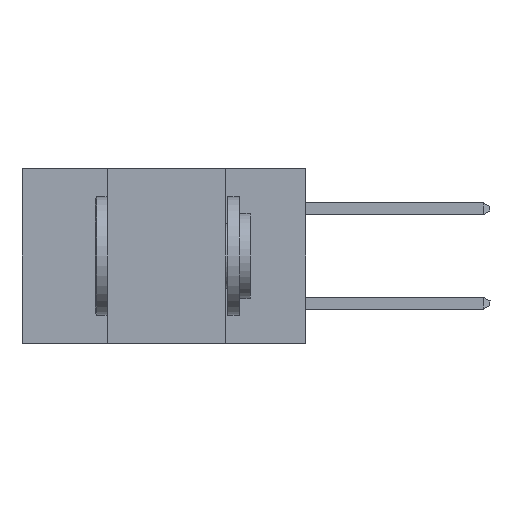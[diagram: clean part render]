
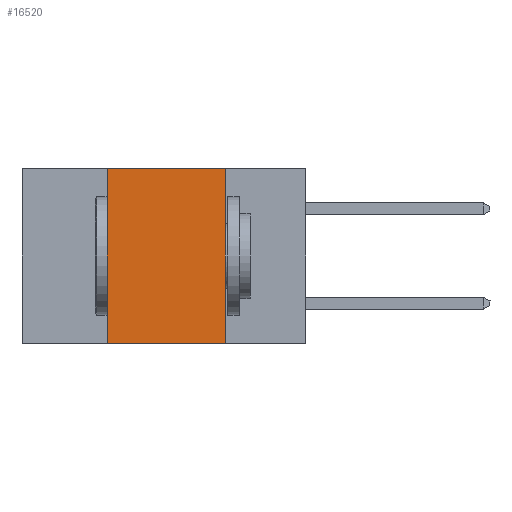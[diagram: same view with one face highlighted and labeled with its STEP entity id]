
A CAD part, left-side view. The second image highlights one B-rep face of the part: STEP entity #16520.
In plain terms, the highlighted planar face has unit normal (-1, 0, 0).
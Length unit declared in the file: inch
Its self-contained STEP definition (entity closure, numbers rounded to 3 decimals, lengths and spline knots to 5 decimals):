
#787 = CARTESIAN_POINT ( 'NONE',  ( 0., 0.42, -0.37 ) ) ;
#958 = CARTESIAN_POINT ( 'NONE',  ( 0., 0.17, 0. ) ) ;
#2046 = ORIENTED_EDGE ( 'NONE', *, *, #6565, .F. ) ;
#2232 = ORIENTED_EDGE ( 'NONE', *, *, #5936, .F. ) ;
#3560 = CARTESIAN_POINT ( 'NONE',  ( 0., 0.42, 0. ) ) ;
#4858 = PLANE ( 'NONE',  #14725 ) ;
#5349 = CARTESIAN_POINT ( 'NONE',  ( 0., 0.42, 0. ) ) ;
#5936 = EDGE_CURVE ( 'NONE', #12882, #23363, #23306, .T. ) ;
#6531 = LINE ( 'NONE', #11302, #21304 ) ;
#6565 = EDGE_CURVE ( 'NONE', #18357, #12882, #14604, .T. ) ;
#6806 = DIRECTION ( 'NONE',  ( 0., 0., -1. ) ) ;
#7772 = FACE_OUTER_BOUND ( 'NONE', #8509, .T. ) ;
#7858 = CARTESIAN_POINT ( 'NONE',  ( 0., 0.17, 0. ) ) ;
#8509 = EDGE_LOOP ( 'NONE', ( #19569, #2232, #2046, #10032 ) ) ;
#8888 = VECTOR ( 'NONE', #15157, 39.37008 ) ;
#9199 = EDGE_CURVE ( 'NONE', #23363, #20766, #16560, .T. ) ;
#10032 = ORIENTED_EDGE ( 'NONE', *, *, #16138, .T. ) ;
#11302 = CARTESIAN_POINT ( 'NONE',  ( 0., 0.6, -0.37 ) ) ;
#12882 = VERTEX_POINT ( 'NONE', #5349 ) ;
#13104 = VECTOR ( 'NONE', #24288, 39.37008 ) ;
#14508 = CARTESIAN_POINT ( 'NONE',  ( 0., 0.6, 0. ) ) ;
#14604 = LINE ( 'NONE', #3560, #8888 ) ;
#14678 = CARTESIAN_POINT ( 'NONE',  ( 0., 0.6, 0. ) ) ;
#14725 = AXIS2_PLACEMENT_3D ( 'NONE', #14508, #18358, #6806 ) ;
#15157 = DIRECTION ( 'NONE',  ( 0., 0., 1. ) ) ;
#16138 = EDGE_CURVE ( 'NONE', #18357, #20766, #6531, .T. ) ;
#16520 = ADVANCED_FACE ( 'NONE', ( #7772 ), #4858, .F. ) ;
#16560 = LINE ( 'NONE', #7858, #21045 ) ;
#18357 = VERTEX_POINT ( 'NONE', #787 ) ;
#18358 = DIRECTION ( 'NONE',  ( 1., 0., 0. ) ) ;
#19569 = ORIENTED_EDGE ( 'NONE', *, *, #9199, .F. ) ;
#20766 = VERTEX_POINT ( 'NONE', #21488 ) ;
#21045 = VECTOR ( 'NONE', #23179, 39.37008 ) ;
#21054 = DIRECTION ( 'NONE',  ( 0., -1., 0. ) ) ;
#21304 = VECTOR ( 'NONE', #21054, 39.37008 ) ;
#21488 = CARTESIAN_POINT ( 'NONE',  ( 0., 0.17, -0.37 ) ) ;
#23179 = DIRECTION ( 'NONE',  ( 0., 0., -1. ) ) ;
#23306 = LINE ( 'NONE', #14678, #13104 ) ;
#23363 = VERTEX_POINT ( 'NONE', #958 ) ;
#24288 = DIRECTION ( 'NONE',  ( 0., -1., 0. ) ) ;
